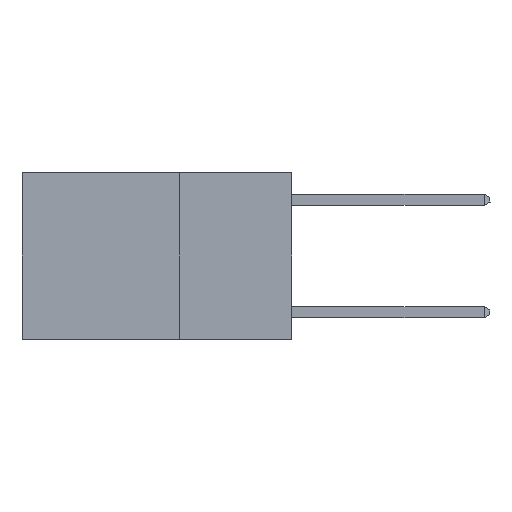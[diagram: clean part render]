
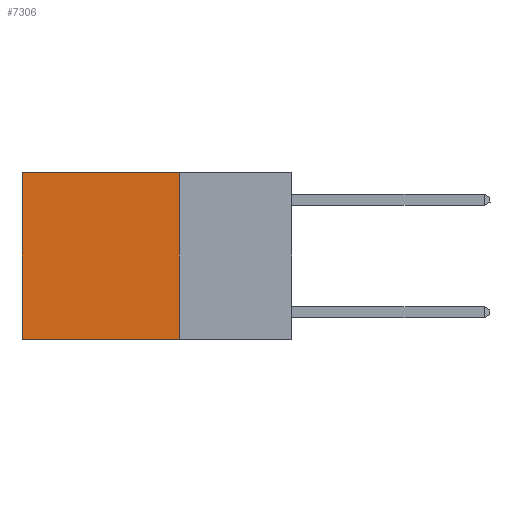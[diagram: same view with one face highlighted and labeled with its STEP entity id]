
A CAD part, left-side view. The second image highlights one B-rep face of the part: STEP entity #7306.
In plain terms, the highlighted planar face has unit normal (-1, 0, 0).
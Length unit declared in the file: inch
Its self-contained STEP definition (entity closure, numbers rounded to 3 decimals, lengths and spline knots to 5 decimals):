
#109 = DIRECTION ( 'NONE',  ( 0., 0., -1. ) ) ;
#251 = EDGE_CURVE ( 'NONE', #927, #6595, #3176, .T. ) ;
#777 = EDGE_CURVE ( 'NONE', #4562, #2418, #3524, .T. ) ;
#895 = EDGE_CURVE ( 'NONE', #2418, #6595, #7510, .T. ) ;
#927 = VERTEX_POINT ( 'NONE', #7021 ) ;
#1283 = ORIENTED_EDGE ( 'NONE', *, *, #4219, .F. ) ;
#1403 = PLANE ( 'NONE',  #2371 ) ;
#2222 = ORIENTED_EDGE ( 'NONE', *, *, #777, .T. ) ;
#2322 = LINE ( 'NONE', #10147, #5569 ) ;
#2371 = AXIS2_PLACEMENT_3D ( 'NONE', #9365, #8481, #5349 ) ;
#2418 = VERTEX_POINT ( 'NONE', #9499 ) ;
#2662 = ORIENTED_EDGE ( 'NONE', *, *, #895, .T. ) ;
#2938 = DIRECTION ( 'NONE',  ( 0., 0., -1. ) ) ;
#3176 = LINE ( 'NONE', #7536, #9647 ) ;
#3524 = LINE ( 'NONE', #8396, #7260 ) ;
#4219 = EDGE_CURVE ( 'NONE', #4562, #927, #2322, .T. ) ;
#4523 = DIRECTION ( 'NONE',  ( 0., 1., 0. ) ) ;
#4562 = VERTEX_POINT ( 'NONE', #10205 ) ;
#5349 = DIRECTION ( 'NONE',  ( 0., 0., -1. ) ) ;
#5569 = VECTOR ( 'NONE', #109, 39.37008 ) ;
#5880 = DIRECTION ( 'NONE',  ( 0., 1., 0. ) ) ;
#6001 = CARTESIAN_POINT ( 'NONE',  ( 0.2625, 0.6, 0. ) ) ;
#6045 = FACE_OUTER_BOUND ( 'NONE', #8703, .T. ) ;
#6584 = CARTESIAN_POINT ( 'NONE',  ( 0.2625, 0.6, -0.37 ) ) ;
#6595 = VERTEX_POINT ( 'NONE', #6584 ) ;
#7021 = CARTESIAN_POINT ( 'NONE',  ( 0.2625, 0.25, -0.37 ) ) ;
#7260 = VECTOR ( 'NONE', #4523, 39.37008 ) ;
#7306 = ADVANCED_FACE ( 'NONE', ( #6045 ), #1403, .F. ) ;
#7389 = VECTOR ( 'NONE', #2938, 39.37008 ) ;
#7510 = LINE ( 'NONE', #6001, #7389 ) ;
#7536 = CARTESIAN_POINT ( 'NONE',  ( 0.2625, 0.25, -0.37 ) ) ;
#8396 = CARTESIAN_POINT ( 'NONE',  ( 0.2625, 0.25, 0. ) ) ;
#8481 = DIRECTION ( 'NONE',  ( 1., 0., 0. ) ) ;
#8703 = EDGE_LOOP ( 'NONE', ( #2662, #10100, #1283, #2222 ) ) ;
#9365 = CARTESIAN_POINT ( 'NONE',  ( 0.2625, 0.25, 0. ) ) ;
#9499 = CARTESIAN_POINT ( 'NONE',  ( 0.2625, 0.6, 0. ) ) ;
#9647 = VECTOR ( 'NONE', #5880, 39.37008 ) ;
#10100 = ORIENTED_EDGE ( 'NONE', *, *, #251, .F. ) ;
#10147 = CARTESIAN_POINT ( 'NONE',  ( 0.2625, 0.25, 0. ) ) ;
#10205 = CARTESIAN_POINT ( 'NONE',  ( 0.2625, 0.25, 0. ) ) ;
